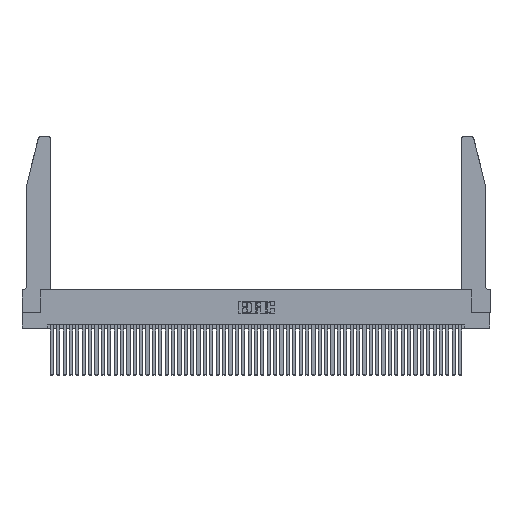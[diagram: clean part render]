
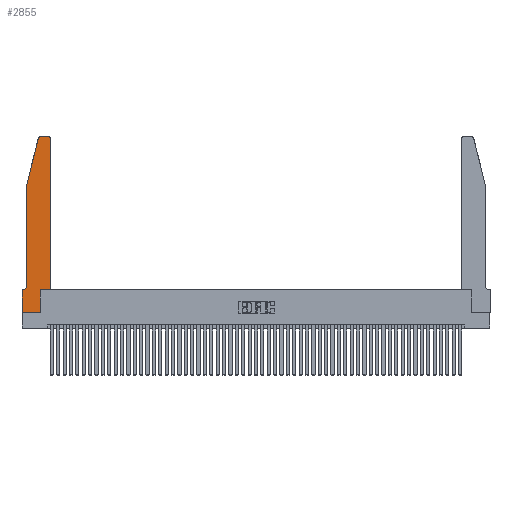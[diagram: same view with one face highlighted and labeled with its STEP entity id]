
A CAD part, top view. The second image highlights one B-rep face of the part: STEP entity #2855.
In plain terms, the highlighted planar face has unit normal (0, 0, 1).
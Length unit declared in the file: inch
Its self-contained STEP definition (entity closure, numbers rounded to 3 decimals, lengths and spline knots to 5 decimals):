
#893 = AXIS2_PLACEMENT_3D ( 'NONE', #5001, #13104, #37589 ) ;
#1359 = EDGE_CURVE ( 'NONE', #24902, #7298, #37708, .T. ) ;
#2406 = ORIENTED_EDGE ( 'NONE', *, *, #42537, .T. ) ;
#2855 = ADVANCED_FACE ( 'NONE', ( #4608 ), #16188, .T. ) ;
#3314 = AXIS2_PLACEMENT_3D ( 'NONE', #46391, #37867, #34297 ) ;
#3588 = VERTEX_POINT ( 'NONE', #11856 ) ;
#3616 = EDGE_CURVE ( 'NONE', #31283, #24902, #43144, .T. ) ;
#4034 = VERTEX_POINT ( 'NONE', #29306 ) ;
#4463 = DIRECTION ( 'NONE',  ( -1., 0., 0. ) ) ;
#4585 = CARTESIAN_POINT ( 'NONE',  ( 0.25487, 2.72718, 0.37 ) ) ;
#4608 = FACE_OUTER_BOUND ( 'NONE', #29531, .T. ) ;
#4745 = DIRECTION ( 'NONE',  ( 0., 0., 1. ) ) ;
#4902 = EDGE_CURVE ( 'NONE', #23175, #3588, #10742, .T. ) ;
#5001 = CARTESIAN_POINT ( 'NONE',  ( 0.0055, 0.42, 0.37 ) ) ;
#5031 = CARTESIAN_POINT ( 'NONE',  ( 0.4205, 2.75, 0.37 ) ) ;
#5844 = CARTESIAN_POINT ( 'NONE',  ( 0.0755, 2., 0.37 ) ) ;
#7298 = VERTEX_POINT ( 'NONE', #42778 ) ;
#8003 = CARTESIAN_POINT ( 'NONE',  ( 0.0755, 2., 0.37 ) ) ;
#8965 = VERTEX_POINT ( 'NONE', #9422 ) ;
#9267 = DIRECTION ( 'NONE',  ( 0., -1., 0. ) ) ;
#9422 = CARTESIAN_POINT ( 'NONE',  ( 0.4505, 2.72, 0.37 ) ) ;
#9564 = DIRECTION ( 'NONE',  ( 1., 0., 0. ) ) ;
#9794 = AXIS2_PLACEMENT_3D ( 'NONE', #36977, #4745, #37345 ) ;
#10742 = LINE ( 'NONE', #34552, #45046 ) ;
#11095 = CARTESIAN_POINT ( 'NONE',  ( 0.4205, 2.72, 0.37 ) ) ;
#11353 = EDGE_CURVE ( 'NONE', #34903, #16876, #40666, .T. ) ;
#11436 = EDGE_CURVE ( 'NONE', #7298, #23407, #38125, .T. ) ;
#11856 = CARTESIAN_POINT ( 'NONE',  ( 0.284, 2.75, 0.37 ) ) ;
#12354 = ORIENTED_EDGE ( 'NONE', *, *, #24863, .T. ) ;
#12636 = CARTESIAN_POINT ( 'NONE',  ( 0.2865, 0.35, 0.37 ) ) ;
#13104 = DIRECTION ( 'NONE',  ( 0., 0., -1. ) ) ;
#14573 = VECTOR ( 'NONE', #28169, 39.37008 ) ;
#15949 = VERTEX_POINT ( 'NONE', #20263 ) ;
#16188 = PLANE ( 'NONE',  #9794 ) ;
#16827 = ORIENTED_EDGE ( 'NONE', *, *, #3616, .T. ) ;
#16837 = CARTESIAN_POINT ( 'NONE',  ( 0.0055, 0.35, 0.37 ) ) ;
#16876 = VERTEX_POINT ( 'NONE', #16837 ) ;
#16902 = CIRCLE ( 'NONE', #42192, 0.03 ) ;
#16999 = LINE ( 'NONE', #8003, #48157 ) ;
#17209 = CARTESIAN_POINT ( 'NONE',  ( 0., 0., 0.37 ) ) ;
#17503 = DIRECTION ( 'NONE',  ( 0., 1., 0. ) ) ;
#17730 = EDGE_CURVE ( 'NONE', #8965, #23175, #16902, .T. ) ;
#18196 = DIRECTION ( 'NONE',  ( 0., -1., 0. ) ) ;
#18212 = DIRECTION ( 'NONE',  ( -1., 0., 0. ) ) ;
#18488 = EDGE_CURVE ( 'NONE', #4034, #31283, #32085, .T. ) ;
#19434 = DIRECTION ( 'NONE',  ( 0., 1., 0. ) ) ;
#19627 = EDGE_CURVE ( 'NONE', #15949, #34903, #23067, .T. ) ;
#19739 = ORIENTED_EDGE ( 'NONE', *, *, #32722, .T. ) ;
#20263 = CARTESIAN_POINT ( 'NONE',  ( 0.0755, 2., 0.37 ) ) ;
#20319 = ORIENTED_EDGE ( 'NONE', *, *, #22746, .T. ) ;
#22081 = CARTESIAN_POINT ( 'NONE',  ( 0., 0., 0.37 ) ) ;
#22746 = EDGE_CURVE ( 'NONE', #16876, #4034, #49007, .T. ) ;
#23067 = LINE ( 'NONE', #5844, #37055 ) ;
#23119 = DIRECTION ( 'NONE',  ( 1., 0., 0. ) ) ;
#23175 = VERTEX_POINT ( 'NONE', #5031 ) ;
#23407 = VERTEX_POINT ( 'NONE', #34571 ) ;
#23457 = VECTOR ( 'NONE', #9564, 39.37008 ) ;
#24592 = CARTESIAN_POINT ( 'NONE',  ( 0.0755, 0.35, 0.37 ) ) ;
#24863 = EDGE_CURVE ( 'NONE', #36007, #15949, #16999, .T. ) ;
#24902 = VERTEX_POINT ( 'NONE', #27477 ) ;
#25783 = ORIENTED_EDGE ( 'NONE', *, *, #19627, .T. ) ;
#26599 = ORIENTED_EDGE ( 'NONE', *, *, #1359, .T. ) ;
#27477 = CARTESIAN_POINT ( 'NONE',  ( 0.2865, 0., 0.37 ) ) ;
#27530 = VECTOR ( 'NONE', #17503, 39.37008 ) ;
#28169 = DIRECTION ( 'NONE',  ( 1., 0., 0. ) ) ;
#29306 = CARTESIAN_POINT ( 'NONE',  ( 0., 0.35, 0.37 ) ) ;
#29531 = EDGE_LOOP ( 'NONE', ( #44041, #2406, #12354, #25783, #42507, #20319, #30960, #16827, #26599, #36296, #19739, #47646 ) ) ;
#30960 = ORIENTED_EDGE ( 'NONE', *, *, #18488, .T. ) ;
#31283 = VERTEX_POINT ( 'NONE', #22081 ) ;
#32085 = LINE ( 'NONE', #17209, #35256 ) ;
#32722 = EDGE_CURVE ( 'NONE', #23407, #8965, #46699, .T. ) ;
#34174 = CARTESIAN_POINT ( 'NONE',  ( 0.0755, 0.42, 0.37 ) ) ;
#34297 = DIRECTION ( 'NONE',  ( 1., 0., 0. ) ) ;
#34552 = CARTESIAN_POINT ( 'NONE',  ( 0.2605, 2.75, 0.37 ) ) ;
#34571 = CARTESIAN_POINT ( 'NONE',  ( 0.4505, 0.35, 0.37 ) ) ;
#34903 = VERTEX_POINT ( 'NONE', #34174 ) ;
#35032 = DIRECTION ( 'NONE',  ( 0., 0., 1. ) ) ;
#35256 = VECTOR ( 'NONE', #9267, 39.37008 ) ;
#35662 = DIRECTION ( 'NONE',  ( -0.239, -0.971, 0. ) ) ;
#35801 = CARTESIAN_POINT ( 'NONE',  ( 0.4505, 0.35, 0.37 ) ) ;
#35870 = VECTOR ( 'NONE', #19434, 39.37008 ) ;
#36007 = VERTEX_POINT ( 'NONE', #4585 ) ;
#36296 = ORIENTED_EDGE ( 'NONE', *, *, #11436, .T. ) ;
#36977 = CARTESIAN_POINT ( 'NONE',  ( 0., 0.35, 0.37 ) ) ;
#37055 = VECTOR ( 'NONE', #18196, 39.37008 ) ;
#37345 = DIRECTION ( 'NONE',  ( 1., 0., 0. ) ) ;
#37589 = DIRECTION ( 'NONE',  ( -1., 0., 0. ) ) ;
#37708 = LINE ( 'NONE', #12636, #27530 ) ;
#37867 = DIRECTION ( 'NONE',  ( 0., 0., 1. ) ) ;
#38125 = LINE ( 'NONE', #46460, #23457 ) ;
#38204 = VECTOR ( 'NONE', #4463, 39.37008 ) ;
#40666 = CIRCLE ( 'NONE', #893, 0.07 ) ;
#42192 = AXIS2_PLACEMENT_3D ( 'NONE', #11095, #35032, #23119 ) ;
#42507 = ORIENTED_EDGE ( 'NONE', *, *, #11353, .T. ) ;
#42537 = EDGE_CURVE ( 'NONE', #3588, #36007, #43705, .T. ) ;
#42778 = CARTESIAN_POINT ( 'NONE',  ( 0.2865, 0.35, 0.37 ) ) ;
#43144 = LINE ( 'NONE', #48089, #14573 ) ;
#43705 = CIRCLE ( 'NONE', #3314, 0.03 ) ;
#44041 = ORIENTED_EDGE ( 'NONE', *, *, #4902, .T. ) ;
#45046 = VECTOR ( 'NONE', #18212, 39.37008 ) ;
#46391 = CARTESIAN_POINT ( 'NONE',  ( 0.284, 2.72, 0.37 ) ) ;
#46460 = CARTESIAN_POINT ( 'NONE',  ( 0.4505, 0.35, 0.37 ) ) ;
#46699 = LINE ( 'NONE', #35801, #35870 ) ;
#47646 = ORIENTED_EDGE ( 'NONE', *, *, #17730, .T. ) ;
#48089 = CARTESIAN_POINT ( 'NONE',  ( 0., 0., 0.37 ) ) ;
#48157 = VECTOR ( 'NONE', #35662, 39.37008 ) ;
#49007 = LINE ( 'NONE', #24592, #38204 ) ;
